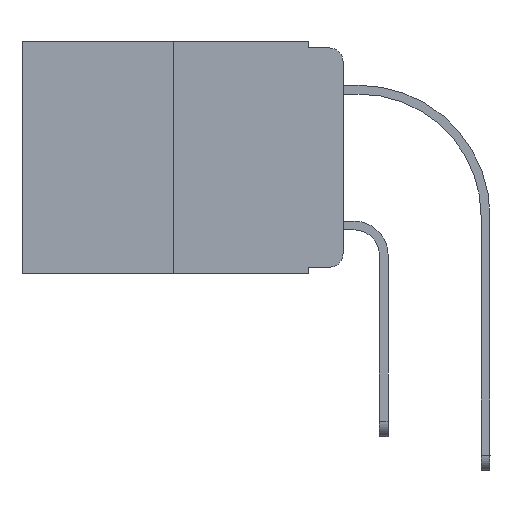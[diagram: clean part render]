
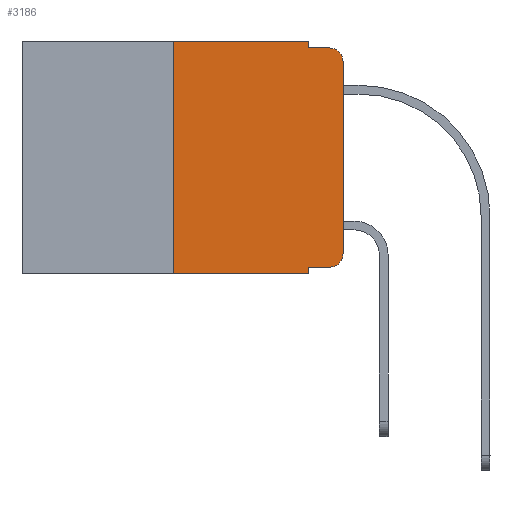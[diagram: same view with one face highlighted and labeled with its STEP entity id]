
A CAD part, left-side view. The second image highlights one B-rep face of the part: STEP entity #3186.
In plain terms, the highlighted planar face has unit normal (-1, 0, 0).
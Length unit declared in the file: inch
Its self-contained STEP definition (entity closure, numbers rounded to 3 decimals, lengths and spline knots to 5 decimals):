
#15 = LINE ( 'NONE', #13469, #4317 ) ;
#172 = VECTOR ( 'NONE', #9666, 39.37008 ) ;
#645 = CARTESIAN_POINT ( 'NONE',  ( 0., 0.051, 0. ) ) ;
#723 = EDGE_CURVE ( 'NONE', #3303, #8135, #14750, .T. ) ;
#780 = CARTESIAN_POINT ( 'NONE',  ( 0., 0., -0.03 ) ) ;
#899 = CARTESIAN_POINT ( 'NONE',  ( 0., 0.25, 0. ) ) ;
#902 = VERTEX_POINT ( 'NONE', #11628 ) ;
#988 = EDGE_CURVE ( 'NONE', #10919, #902, #14176, .T. ) ;
#1187 = CARTESIAN_POINT ( 'NONE',  ( 0., 0.051, -0.01 ) ) ;
#1375 = ORIENTED_EDGE ( 'NONE', *, *, #10261, .T. ) ;
#1446 = DIRECTION ( 'NONE',  ( -1., 0., 0. ) ) ;
#1557 = EDGE_CURVE ( 'NONE', #3303, #8589, #8882, .T. ) ;
#1871 = VERTEX_POINT ( 'NONE', #8408 ) ;
#2202 = CARTESIAN_POINT ( 'NONE',  ( 0., 0.25, -0.343 ) ) ;
#2221 = DIRECTION ( 'NONE',  ( 0., 0., 1. ) ) ;
#2269 = DIRECTION ( 'NONE',  ( 0., 0., -1. ) ) ;
#2292 = CIRCLE ( 'NONE', #10412, 0.02 ) ;
#2456 = CARTESIAN_POINT ( 'NONE',  ( 0., 0.051, 0. ) ) ;
#2675 = DIRECTION ( 'NONE',  ( 1., 0., 0. ) ) ;
#2896 = LINE ( 'NONE', #11636, #13738 ) ;
#3018 = VERTEX_POINT ( 'NONE', #9459 ) ;
#3186 = ADVANCED_FACE ( 'NONE', ( #14777 ), #10004, .F. ) ;
#3303 = VERTEX_POINT ( 'NONE', #2202 ) ;
#3593 = ORIENTED_EDGE ( 'NONE', *, *, #7402, .T. ) ;
#3703 = EDGE_CURVE ( 'NONE', #8589, #10919, #2896, .T. ) ;
#3809 = DIRECTION ( 'NONE',  ( 0., 0., -1. ) ) ;
#3822 = VECTOR ( 'NONE', #13725, 39.37008 ) ;
#3857 = CARTESIAN_POINT ( 'NONE',  ( 0., 0.473, -0.343 ) ) ;
#4279 = EDGE_CURVE ( 'NONE', #9110, #9369, #13109, .T. ) ;
#4317 = VECTOR ( 'NONE', #2269, 39.37008 ) ;
#4341 = DIRECTION ( 'NONE',  ( 0., -1., 0. ) ) ;
#4412 = LINE ( 'NONE', #9495, #7525 ) ;
#4535 = CARTESIAN_POINT ( 'NONE',  ( 0., 0.051, -0.343 ) ) ;
#4592 = DIRECTION ( 'NONE',  ( -1., 0., 0. ) ) ;
#4832 = CARTESIAN_POINT ( 'NONE',  ( 0., 0.02, -0.313 ) ) ;
#4841 = ORIENTED_EDGE ( 'NONE', *, *, #988, .F. ) ;
#6236 = CIRCLE ( 'NONE', #8048, 0.02 ) ;
#6997 = DIRECTION ( 'NONE',  ( 0., -1., 0. ) ) ;
#7319 = EDGE_CURVE ( 'NONE', #3018, #8135, #15, .T. ) ;
#7402 = EDGE_CURVE ( 'NONE', #9369, #1871, #2292, .T. ) ;
#7525 = VECTOR ( 'NONE', #6997, 39.37008 ) ;
#8048 = AXIS2_PLACEMENT_3D ( 'NONE', #4832, #4592, #14356 ) ;
#8135 = VERTEX_POINT ( 'NONE', #4535 ) ;
#8408 = CARTESIAN_POINT ( 'NONE',  ( 0., 0.02, -0.01 ) ) ;
#8589 = VERTEX_POINT ( 'NONE', #899 ) ;
#8882 = LINE ( 'NONE', #12524, #3822 ) ;
#9110 = VERTEX_POINT ( 'NONE', #14648 ) ;
#9310 = ORIENTED_EDGE ( 'NONE', *, *, #12847, .F. ) ;
#9369 = VERTEX_POINT ( 'NONE', #780 ) ;
#9459 = CARTESIAN_POINT ( 'NONE',  ( 0., 0.051, -0.333 ) ) ;
#9480 = ORIENTED_EDGE ( 'NONE', *, *, #1557, .F. ) ;
#9495 = CARTESIAN_POINT ( 'NONE',  ( 0., 0.051, -0.333 ) ) ;
#9666 = DIRECTION ( 'NONE',  ( 0., -1., 0. ) ) ;
#10004 = PLANE ( 'NONE',  #10437 ) ;
#10081 = DIRECTION ( 'NONE',  ( 0., -1., 0. ) ) ;
#10261 = EDGE_CURVE ( 'NONE', #3018, #12470, #4412, .T. ) ;
#10412 = AXIS2_PLACEMENT_3D ( 'NONE', #15647, #1446, #12498 ) ;
#10437 = AXIS2_PLACEMENT_3D ( 'NONE', #13575, #2675, #3809 ) ;
#10919 = VERTEX_POINT ( 'NONE', #2456 ) ;
#10985 = EDGE_LOOP ( 'NONE', ( #12012, #3593, #9310, #4841, #13340, #9480, #11281, #14240, #1375, #14595 ) ) ;
#11281 = ORIENTED_EDGE ( 'NONE', *, *, #723, .T. ) ;
#11628 = CARTESIAN_POINT ( 'NONE',  ( 0., 0.051, -0.01 ) ) ;
#11636 = CARTESIAN_POINT ( 'NONE',  ( 0., 0.473, 0. ) ) ;
#11730 = VECTOR ( 'NONE', #15469, 39.37008 ) ;
#12012 = ORIENTED_EDGE ( 'NONE', *, *, #4279, .T. ) ;
#12470 = VERTEX_POINT ( 'NONE', #14820 ) ;
#12498 = DIRECTION ( 'NONE',  ( 0., 0., -1. ) ) ;
#12524 = CARTESIAN_POINT ( 'NONE',  ( 0., 0.25, 0. ) ) ;
#12736 = VECTOR ( 'NONE', #2221, 39.37008 ) ;
#12847 = EDGE_CURVE ( 'NONE', #902, #1871, #14856, .T. ) ;
#12920 = VECTOR ( 'NONE', #10081, 39.37008 ) ;
#13109 = LINE ( 'NONE', #13197, #12736 ) ;
#13197 = CARTESIAN_POINT ( 'NONE',  ( 0., 0., 0. ) ) ;
#13340 = ORIENTED_EDGE ( 'NONE', *, *, #3703, .F. ) ;
#13469 = CARTESIAN_POINT ( 'NONE',  ( 0., 0.051, 0. ) ) ;
#13575 = CARTESIAN_POINT ( 'NONE',  ( 0., 0.473, 0. ) ) ;
#13725 = DIRECTION ( 'NONE',  ( 0., 0., 1. ) ) ;
#13738 = VECTOR ( 'NONE', #4341, 39.37008 ) ;
#14176 = LINE ( 'NONE', #645, #11730 ) ;
#14240 = ORIENTED_EDGE ( 'NONE', *, *, #7319, .F. ) ;
#14356 = DIRECTION ( 'NONE',  ( 0., 0., -1. ) ) ;
#14595 = ORIENTED_EDGE ( 'NONE', *, *, #14887, .T. ) ;
#14648 = CARTESIAN_POINT ( 'NONE',  ( 0., 0., -0.313 ) ) ;
#14750 = LINE ( 'NONE', #3857, #172 ) ;
#14777 = FACE_OUTER_BOUND ( 'NONE', #10985, .T. ) ;
#14820 = CARTESIAN_POINT ( 'NONE',  ( 0., 0.02, -0.333 ) ) ;
#14856 = LINE ( 'NONE', #1187, #12920 ) ;
#14887 = EDGE_CURVE ( 'NONE', #12470, #9110, #6236, .T. ) ;
#15469 = DIRECTION ( 'NONE',  ( 0., 0., -1. ) ) ;
#15647 = CARTESIAN_POINT ( 'NONE',  ( 0., 0.02, -0.03 ) ) ;
